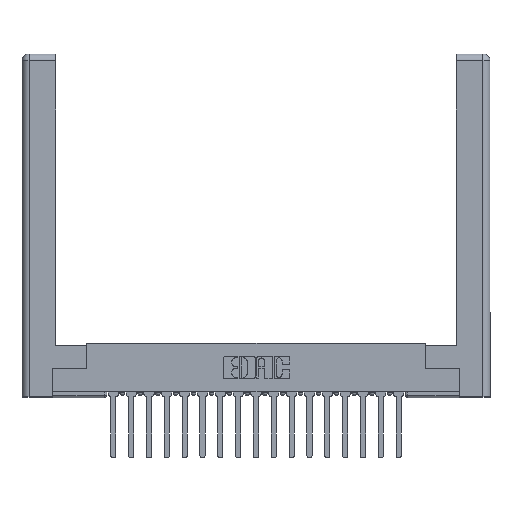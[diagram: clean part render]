
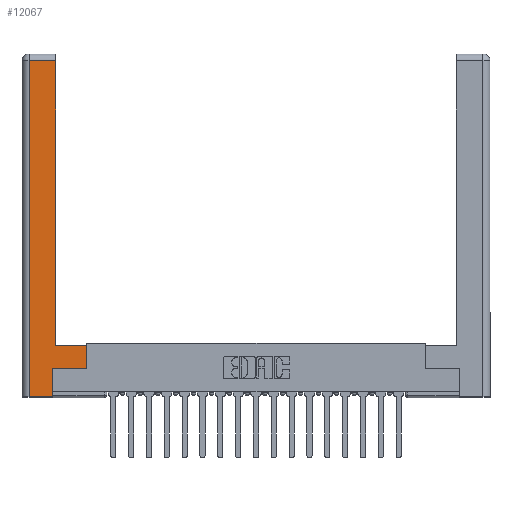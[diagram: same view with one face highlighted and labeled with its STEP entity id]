
A CAD part, top view. The second image highlights one B-rep face of the part: STEP entity #12067.
In plain terms, the highlighted planar face has unit normal (0, 0, 1).
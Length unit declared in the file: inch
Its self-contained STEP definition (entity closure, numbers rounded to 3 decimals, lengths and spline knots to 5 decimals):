
#348 = CARTESIAN_POINT ( 'NONE',  ( 0.295, 3., 0. ) ) ;
#567 = ORIENTED_EDGE ( 'NONE', *, *, #18795, .T. ) ;
#674 = VERTEX_POINT ( 'NONE', #8313 ) ;
#680 = CARTESIAN_POINT ( 'NONE',  ( 0.0615, 2.94, 0. ) ) ;
#1050 = ORIENTED_EDGE ( 'NONE', *, *, #18319, .T. ) ;
#1238 = DIRECTION ( 'NONE',  ( 0., -1., 0. ) ) ;
#1341 = CARTESIAN_POINT ( 'NONE',  ( 0.0615, 0., 0. ) ) ;
#1660 = CARTESIAN_POINT ( 'NONE',  ( 0.565, 0.45, 0. ) ) ;
#1906 = LINE ( 'NONE', #680, #17514 ) ;
#2026 = DIRECTION ( 'NONE',  ( -1., 0., 0. ) ) ;
#2090 = DIRECTION ( 'NONE',  ( 0., 1., 0. ) ) ;
#3474 = EDGE_CURVE ( 'NONE', #4760, #19570, #1906, .T. ) ;
#3666 = VECTOR ( 'NONE', #2026, 39.37008 ) ;
#3706 = CARTESIAN_POINT ( 'NONE',  ( 0.265, 0., 0. ) ) ;
#4091 = CARTESIAN_POINT ( 'NONE',  ( 0., 0., 0. ) ) ;
#4217 = LINE ( 'NONE', #5842, #9435 ) ;
#4286 = VECTOR ( 'NONE', #11970, 39.37008 ) ;
#4501 = ORIENTED_EDGE ( 'NONE', *, *, #5909, .T. ) ;
#4503 = CARTESIAN_POINT ( 'NONE',  ( 0.295, 0.45, 0. ) ) ;
#4760 = VERTEX_POINT ( 'NONE', #11629 ) ;
#5815 = DIRECTION ( 'NONE',  ( 0., 0., -1. ) ) ;
#5842 = CARTESIAN_POINT ( 'NONE',  ( 0.565, 0.45, 0. ) ) ;
#5909 = EDGE_CURVE ( 'NONE', #19570, #16572, #12380, .T. ) ;
#8243 = DIRECTION ( 'NONE',  ( -1., 0., 0. ) ) ;
#8313 = CARTESIAN_POINT ( 'NONE',  ( 0.565, 0.245, 0. ) ) ;
#8328 = CARTESIAN_POINT ( 'NONE',  ( 0.265, 0., 0. ) ) ;
#8600 = ORIENTED_EDGE ( 'NONE', *, *, #12966, .T. ) ;
#9032 = ORIENTED_EDGE ( 'NONE', *, *, #15961, .T. ) ;
#9366 = VECTOR ( 'NONE', #14533, 39.37008 ) ;
#9435 = VECTOR ( 'NONE', #13516, 39.37008 ) ;
#9725 = VECTOR ( 'NONE', #10392, 39.37008 ) ;
#10392 = DIRECTION ( 'NONE',  ( 1., 0., 0. ) ) ;
#11629 = CARTESIAN_POINT ( 'NONE',  ( 0.295, 2.94, 0. ) ) ;
#11960 = EDGE_CURVE ( 'NONE', #16572, #19841, #17833, .T. ) ;
#11970 = DIRECTION ( 'NONE',  ( 0., 1., 0. ) ) ;
#12007 = CARTESIAN_POINT ( 'NONE',  ( 0.265, 0.245, 0. ) ) ;
#12043 = ORIENTED_EDGE ( 'NONE', *, *, #19334, .T. ) ;
#12067 = ADVANCED_FACE ( 'NONE', ( #14731 ), #15124, .F. ) ;
#12380 = LINE ( 'NONE', #1341, #17134 ) ;
#12966 = EDGE_CURVE ( 'NONE', #15597, #674, #17991, .T. ) ;
#13204 = CARTESIAN_POINT ( 'NONE',  ( 0.265, 0.245, 0. ) ) ;
#13265 = ORIENTED_EDGE ( 'NONE', *, *, #11960, .T. ) ;
#13503 = LINE ( 'NONE', #13204, #4286 ) ;
#13516 = DIRECTION ( 'NONE',  ( 0., 1., 0. ) ) ;
#13763 = CARTESIAN_POINT ( 'NONE',  ( 0.0615, 2.94, 0. ) ) ;
#14047 = VECTOR ( 'NONE', #2090, 39.37008 ) ;
#14182 = CARTESIAN_POINT ( 'NONE',  ( 0.295, 0.45, 0. ) ) ;
#14533 = DIRECTION ( 'NONE',  ( 1., 0., 0. ) ) ;
#14731 = FACE_OUTER_BOUND ( 'NONE', #16150, .T. ) ;
#14991 = ORIENTED_EDGE ( 'NONE', *, *, #3474, .T. ) ;
#15085 = VERTEX_POINT ( 'NONE', #1660 ) ;
#15124 = PLANE ( 'NONE',  #18195 ) ;
#15597 = VERTEX_POINT ( 'NONE', #12007 ) ;
#15961 = EDGE_CURVE ( 'NONE', #674, #15085, #4217, .T. ) ;
#16034 = LINE ( 'NONE', #14182, #3666 ) ;
#16150 = EDGE_LOOP ( 'NONE', ( #1050, #14991, #4501, #13265, #567, #8600, #9032, #12043 ) ) ;
#16433 = CARTESIAN_POINT ( 'NONE',  ( 0.565, 0.245, 0. ) ) ;
#16572 = VERTEX_POINT ( 'NONE', #19120 ) ;
#17134 = VECTOR ( 'NONE', #1238, 39.37008 ) ;
#17514 = VECTOR ( 'NONE', #8243, 39.37008 ) ;
#17833 = LINE ( 'NONE', #3706, #9366 ) ;
#17991 = LINE ( 'NONE', #16433, #9725 ) ;
#18195 = AXIS2_PLACEMENT_3D ( 'NONE', #4091, #5815, #19582 ) ;
#18319 = EDGE_CURVE ( 'NONE', #18983, #4760, #19205, .T. ) ;
#18795 = EDGE_CURVE ( 'NONE', #19841, #15597, #13503, .T. ) ;
#18983 = VERTEX_POINT ( 'NONE', #4503 ) ;
#19120 = CARTESIAN_POINT ( 'NONE',  ( 0.0615, 0., 0. ) ) ;
#19205 = LINE ( 'NONE', #348, #14047 ) ;
#19334 = EDGE_CURVE ( 'NONE', #15085, #18983, #16034, .T. ) ;
#19570 = VERTEX_POINT ( 'NONE', #13763 ) ;
#19582 = DIRECTION ( 'NONE',  ( -1., 0., 0. ) ) ;
#19841 = VERTEX_POINT ( 'NONE', #8328 ) ;
